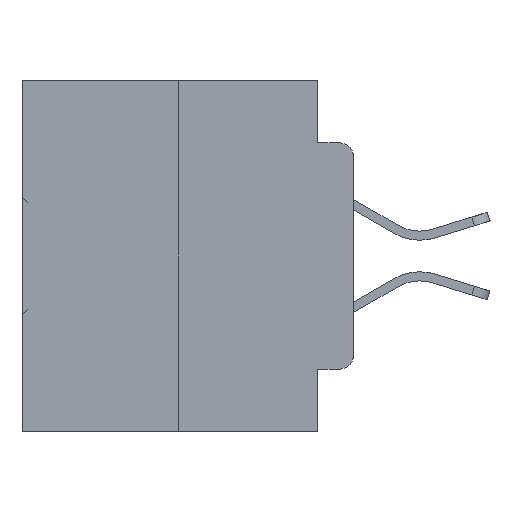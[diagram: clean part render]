
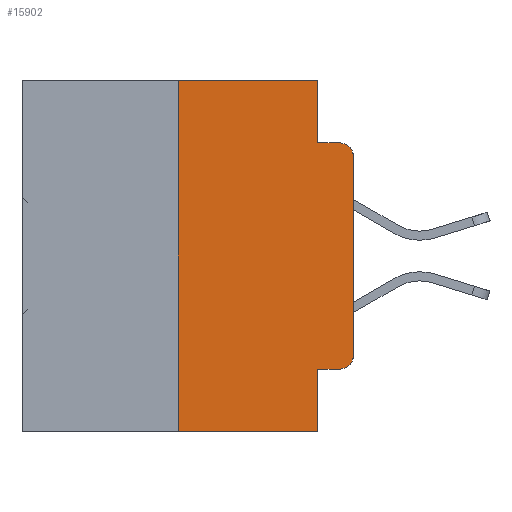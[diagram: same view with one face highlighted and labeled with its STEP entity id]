
A CAD part, left-side view. The second image highlights one B-rep face of the part: STEP entity #15902.
In plain terms, the highlighted planar face has unit normal (-1, 0, 0).
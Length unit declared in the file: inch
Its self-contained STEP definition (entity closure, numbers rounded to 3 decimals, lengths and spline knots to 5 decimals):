
#133 = VECTOR ( 'NONE', #16876, 39.37008 ) ;
#755 = LINE ( 'NONE', #926, #7099 ) ;
#879 = EDGE_CURVE ( 'NONE', #2243, #2585, #28504, .T. ) ;
#926 = CARTESIAN_POINT ( 'NONE',  ( 0., 0.051, -0.0885 ) ) ;
#2243 = VERTEX_POINT ( 'NONE', #17908 ) ;
#2585 = VERTEX_POINT ( 'NONE', #7858 ) ;
#2975 = CARTESIAN_POINT ( 'NONE',  ( 0., 0., -0.3915 ) ) ;
#3241 = VECTOR ( 'NONE', #28620, 39.37008 ) ;
#3490 = CARTESIAN_POINT ( 'NONE',  ( 0., 0.051, -0.4115 ) ) ;
#4968 = LINE ( 'NONE', #5015, #3241 ) ;
#5015 = CARTESIAN_POINT ( 'NONE',  ( 0., 0.473, -0.5 ) ) ;
#6304 = CARTESIAN_POINT ( 'NONE',  ( 0., 0.25, -0.5 ) ) ;
#6661 = VERTEX_POINT ( 'NONE', #14034 ) ;
#6817 = CARTESIAN_POINT ( 'NONE',  ( 0., 0.051, -0.4115 ) ) ;
#7068 = LINE ( 'NONE', #7815, #20264 ) ;
#7099 = VECTOR ( 'NONE', #14917, 39.37008 ) ;
#7815 = CARTESIAN_POINT ( 'NONE',  ( 0., 0.25, 0. ) ) ;
#7858 = CARTESIAN_POINT ( 'NONE',  ( 0., 0.02, -0.0885 ) ) ;
#7927 = LINE ( 'NONE', #13519, #14156 ) ;
#7985 = ORIENTED_EDGE ( 'NONE', *, *, #879, .T. ) ;
#8567 = FACE_OUTER_BOUND ( 'NONE', #19212, .T. ) ;
#9244 = ORIENTED_EDGE ( 'NONE', *, *, #19497, .F. ) ;
#10374 = DIRECTION ( 'NONE',  ( 0., 0., -1. ) ) ;
#11579 = DIRECTION ( 'NONE',  ( 0., -1., 0. ) ) ;
#11866 = CIRCLE ( 'NONE', #18527, 0.02 ) ;
#12296 = EDGE_CURVE ( 'NONE', #15250, #23078, #22366, .T. ) ;
#12548 = EDGE_CURVE ( 'NONE', #23078, #2585, #755, .T. ) ;
#13343 = EDGE_CURVE ( 'NONE', #30351, #31599, #4968, .T. ) ;
#13519 = CARTESIAN_POINT ( 'NONE',  ( 0., 0.473, 0. ) ) ;
#14034 = CARTESIAN_POINT ( 'NONE',  ( 0., 0.02, -0.4115 ) ) ;
#14156 = VECTOR ( 'NONE', #21407, 39.37008 ) ;
#14587 = VECTOR ( 'NONE', #31377, 39.37008 ) ;
#14917 = DIRECTION ( 'NONE',  ( 0., -1., 0. ) ) ;
#15250 = VERTEX_POINT ( 'NONE', #31170 ) ;
#15864 = CARTESIAN_POINT ( 'NONE',  ( 0., 0.02, -0.3915 ) ) ;
#15902 = ADVANCED_FACE ( 'NONE', ( #8567 ), #31082, .F. ) ;
#16685 = ORIENTED_EDGE ( 'NONE', *, *, #12548, .F. ) ;
#16717 = ORIENTED_EDGE ( 'NONE', *, *, #33966, .T. ) ;
#16876 = DIRECTION ( 'NONE',  ( 0., 0., -1. ) ) ;
#16964 = VERTEX_POINT ( 'NONE', #6817 ) ;
#17200 = CARTESIAN_POINT ( 'NONE',  ( 0., 0., 0. ) ) ;
#17306 = LINE ( 'NONE', #17200, #31029 ) ;
#17908 = CARTESIAN_POINT ( 'NONE',  ( 0., 0., -0.1085 ) ) ;
#18512 = DIRECTION ( 'NONE',  ( 0., 0., -1. ) ) ;
#18527 = AXIS2_PLACEMENT_3D ( 'NONE', #15864, #33938, #18512 ) ;
#18567 = LINE ( 'NONE', #3490, #31454 ) ;
#19076 = EDGE_CURVE ( 'NONE', #25113, #15250, #7927, .T. ) ;
#19212 = EDGE_LOOP ( 'NONE', ( #26421, #7985, #16685, #33649, #28464, #9244, #31650, #19583, #28070, #16717 ) ) ;
#19497 = EDGE_CURVE ( 'NONE', #30351, #25113, #7068, .T. ) ;
#19583 = ORIENTED_EDGE ( 'NONE', *, *, #26546, .F. ) ;
#19619 = VERTEX_POINT ( 'NONE', #2975 ) ;
#20264 = VECTOR ( 'NONE', #26016, 39.37008 ) ;
#20509 = LINE ( 'NONE', #32331, #133 ) ;
#20721 = CARTESIAN_POINT ( 'NONE',  ( 0., 0.473, 0. ) ) ;
#21148 = EDGE_CURVE ( 'NONE', #19619, #2243, #17306, .T. ) ;
#21155 = CARTESIAN_POINT ( 'NONE',  ( 0., 0.02, -0.1085 ) ) ;
#21407 = DIRECTION ( 'NONE',  ( 0., -1., 0. ) ) ;
#22366 = LINE ( 'NONE', #28829, #14587 ) ;
#22439 = DIRECTION ( 'NONE',  ( 0., 0., 1. ) ) ;
#23078 = VERTEX_POINT ( 'NONE', #23546 ) ;
#23546 = CARTESIAN_POINT ( 'NONE',  ( 0., 0.051, -0.0885 ) ) ;
#24610 = CARTESIAN_POINT ( 'NONE',  ( 0., 0.051, -0.5 ) ) ;
#25113 = VERTEX_POINT ( 'NONE', #28752 ) ;
#25909 = AXIS2_PLACEMENT_3D ( 'NONE', #21155, #30541, #29204 ) ;
#26016 = DIRECTION ( 'NONE',  ( 0., 0., 1. ) ) ;
#26021 = DIRECTION ( 'NONE',  ( 1., 0., 0. ) ) ;
#26421 = ORIENTED_EDGE ( 'NONE', *, *, #21148, .T. ) ;
#26546 = EDGE_CURVE ( 'NONE', #16964, #31599, #20509, .T. ) ;
#27473 = AXIS2_PLACEMENT_3D ( 'NONE', #20721, #26021, #10374 ) ;
#28070 = ORIENTED_EDGE ( 'NONE', *, *, #31605, .T. ) ;
#28464 = ORIENTED_EDGE ( 'NONE', *, *, #19076, .F. ) ;
#28504 = CIRCLE ( 'NONE', #25909, 0.02 ) ;
#28620 = DIRECTION ( 'NONE',  ( 0., -1., 0. ) ) ;
#28752 = CARTESIAN_POINT ( 'NONE',  ( 0., 0.25, 0. ) ) ;
#28829 = CARTESIAN_POINT ( 'NONE',  ( 0., 0.051, 0. ) ) ;
#29204 = DIRECTION ( 'NONE',  ( 0., 0., -1. ) ) ;
#30351 = VERTEX_POINT ( 'NONE', #6304 ) ;
#30541 = DIRECTION ( 'NONE',  ( -1., 0., 0. ) ) ;
#31029 = VECTOR ( 'NONE', #22439, 39.37008 ) ;
#31082 = PLANE ( 'NONE',  #27473 ) ;
#31170 = CARTESIAN_POINT ( 'NONE',  ( 0., 0.051, 0. ) ) ;
#31377 = DIRECTION ( 'NONE',  ( 0., 0., -1. ) ) ;
#31454 = VECTOR ( 'NONE', #11579, 39.37008 ) ;
#31599 = VERTEX_POINT ( 'NONE', #24610 ) ;
#31605 = EDGE_CURVE ( 'NONE', #16964, #6661, #18567, .T. ) ;
#31650 = ORIENTED_EDGE ( 'NONE', *, *, #13343, .T. ) ;
#32331 = CARTESIAN_POINT ( 'NONE',  ( 0., 0.051, 0. ) ) ;
#33649 = ORIENTED_EDGE ( 'NONE', *, *, #12296, .F. ) ;
#33938 = DIRECTION ( 'NONE',  ( -1., 0., 0. ) ) ;
#33966 = EDGE_CURVE ( 'NONE', #6661, #19619, #11866, .T. ) ;
